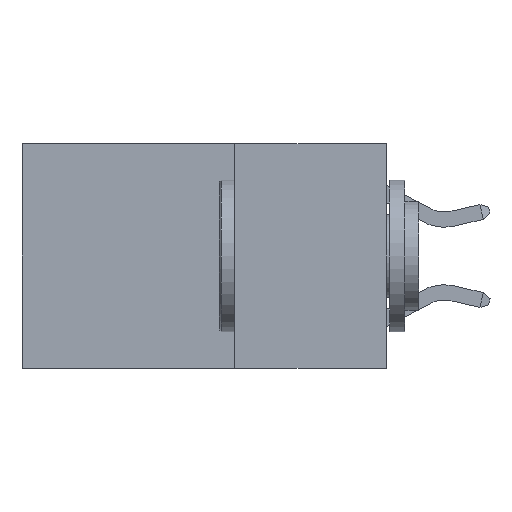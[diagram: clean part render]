
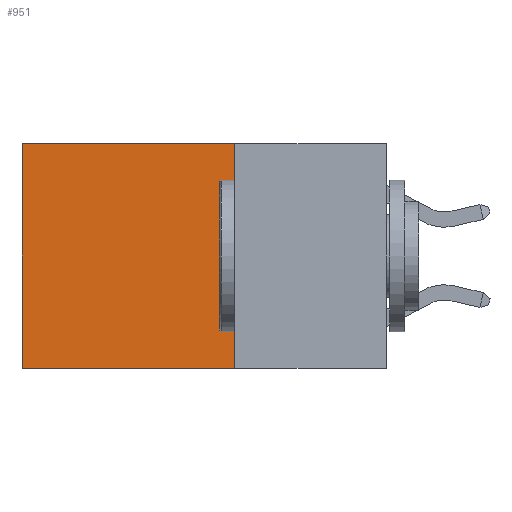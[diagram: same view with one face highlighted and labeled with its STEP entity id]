
A CAD part, left-side view. The second image highlights one B-rep face of the part: STEP entity #951.
In plain terms, the highlighted planar face has unit normal (-1, 0, 0).
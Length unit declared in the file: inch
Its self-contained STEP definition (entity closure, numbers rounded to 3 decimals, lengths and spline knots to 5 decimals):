
#214 = ORIENTED_EDGE ( 'NONE', *, *, #1851, .F. ) ;
#871 = CARTESIAN_POINT ( 'NONE',  ( 0.2625, 0.25, 0. ) ) ;
#951 = ADVANCED_FACE ( 'NONE', ( #9079 ), #8777, .F. ) ;
#1691 = CARTESIAN_POINT ( 'NONE',  ( 0.2625, 0.25, -0.37 ) ) ;
#1851 = EDGE_CURVE ( 'NONE', #3447, #7343, #2257, .T. ) ;
#2257 = LINE ( 'NONE', #11380, #11154 ) ;
#2593 = CARTESIAN_POINT ( 'NONE',  ( 0.2625, 0.6, 0. ) ) ;
#3290 = EDGE_CURVE ( 'NONE', #3447, #8167, #9159, .T. ) ;
#3447 = VERTEX_POINT ( 'NONE', #8883 ) ;
#3508 = CARTESIAN_POINT ( 'NONE',  ( 0.2625, 0.25, 0. ) ) ;
#3827 = LINE ( 'NONE', #6443, #9006 ) ;
#3846 = DIRECTION ( 'NONE',  ( 0., 1., 0. ) ) ;
#4243 = VECTOR ( 'NONE', #6144, 39.37008 ) ;
#4440 = DIRECTION ( 'NONE',  ( 0., 0., -1. ) ) ;
#4599 = EDGE_CURVE ( 'NONE', #8167, #6579, #11109, .T. ) ;
#4770 = ORIENTED_EDGE ( 'NONE', *, *, #4599, .T. ) ;
#4962 = EDGE_CURVE ( 'NONE', #7343, #6579, #3827, .T. ) ;
#5029 = ORIENTED_EDGE ( 'NONE', *, *, #3290, .T. ) ;
#5053 = VECTOR ( 'NONE', #7770, 39.37008 ) ;
#5473 = EDGE_LOOP ( 'NONE', ( #4770, #9370, #214, #5029 ) ) ;
#6144 = DIRECTION ( 'NONE',  ( 0., 1., 0. ) ) ;
#6246 = DIRECTION ( 'NONE',  ( 0., 0., -1. ) ) ;
#6443 = CARTESIAN_POINT ( 'NONE',  ( 0.2625, 0.25, -0.37 ) ) ;
#6579 = VERTEX_POINT ( 'NONE', #9988 ) ;
#7343 = VERTEX_POINT ( 'NONE', #1691 ) ;
#7770 = DIRECTION ( 'NONE',  ( 0., 0., -1. ) ) ;
#8167 = VERTEX_POINT ( 'NONE', #11301 ) ;
#8777 = PLANE ( 'NONE',  #9311 ) ;
#8883 = CARTESIAN_POINT ( 'NONE',  ( 0.2625, 0.25, 0. ) ) ;
#9006 = VECTOR ( 'NONE', #3846, 39.37008 ) ;
#9079 = FACE_OUTER_BOUND ( 'NONE', #5473, .T. ) ;
#9159 = LINE ( 'NONE', #3508, #4243 ) ;
#9311 = AXIS2_PLACEMENT_3D ( 'NONE', #871, #9631, #4440 ) ;
#9370 = ORIENTED_EDGE ( 'NONE', *, *, #4962, .F. ) ;
#9631 = DIRECTION ( 'NONE',  ( 1., 0., 0. ) ) ;
#9988 = CARTESIAN_POINT ( 'NONE',  ( 0.2625, 0.6, -0.37 ) ) ;
#11109 = LINE ( 'NONE', #2593, #5053 ) ;
#11154 = VECTOR ( 'NONE', #6246, 39.37008 ) ;
#11301 = CARTESIAN_POINT ( 'NONE',  ( 0.2625, 0.6, 0. ) ) ;
#11380 = CARTESIAN_POINT ( 'NONE',  ( 0.2625, 0.25, 0. ) ) ;
